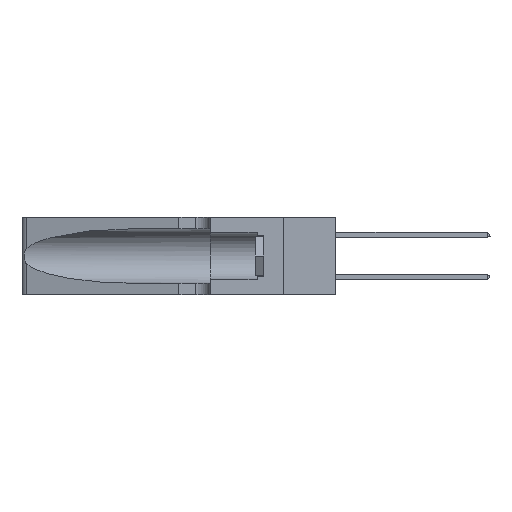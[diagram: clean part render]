
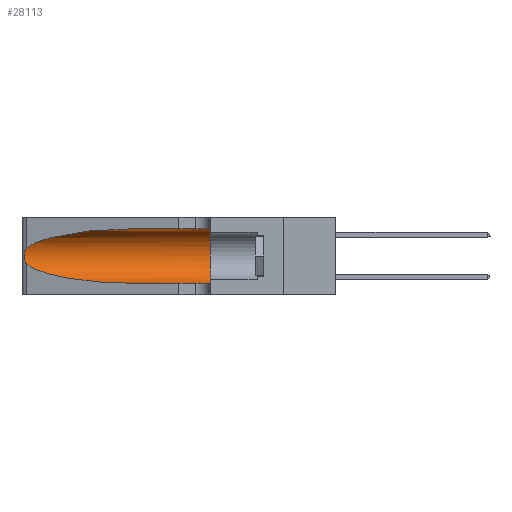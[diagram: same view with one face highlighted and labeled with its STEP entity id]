
A CAD part, left-side view. The second image highlights one B-rep face of the part: STEP entity #28113.
In plain terms, the highlighted cylindrical face has radius 3.308 mm (diameter 6.617 mm), a partial arc.
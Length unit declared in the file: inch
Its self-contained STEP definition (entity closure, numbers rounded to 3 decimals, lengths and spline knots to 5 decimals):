
#178 = CARTESIAN_POINT ( 'NONE',  ( 0.25856, 1.23593, 0.16098 ) ) ;
#697 = CARTESIAN_POINT ( 'NONE',  ( 0.1305, 0.72297, 0.05475 ) ) ;
#1665 = DIRECTION ( 'NONE',  ( 0., -1., 0. ) ) ;
#2849 = CARTESIAN_POINT ( 'NONE',  ( 0.25487, 1.22718, 0.14631 ) ) ;
#4685 = CARTESIAN_POINT ( 'NONE',  ( 0.1305, 0.35, 0.05475 ) ) ;
#5077 = CARTESIAN_POINT ( 'NONE',  ( 0.25639, 1.23186, 0.15144 ) ) ;
#5295 = CARTESIAN_POINT ( 'NONE',  ( 0.26075, 1.23896, 0.19203 ) ) ;
#5450 = ORIENTED_EDGE ( 'NONE', *, *, #28094, .T. ) ;
#5750 = CYLINDRICAL_SURFACE ( 'NONE', #9639, 0.13025 ) ;
#6101 = CARTESIAN_POINT ( 'NONE',  ( 0.25487, 1.22718, 0.22369 ) ) ;
#6136 = CARTESIAN_POINT ( 'NONE',  ( 0.2373, 1.15595, 0.08982 ) ) ;
#7564 = LINE ( 'NONE', #15028, #27845 ) ;
#8656 = DIRECTION ( 'NONE',  ( 0., 0., -1. ) ) ;
#9103 = VERTEX_POINT ( 'NONE', #15913 ) ;
#9639 = AXIS2_PLACEMENT_3D ( 'NONE', #24387, #21619, #8656 ) ;
#9834 = LINE ( 'NONE', #30056, #26365 ) ;
#10285 = VERTEX_POINT ( 'NONE', #33782 ) ;
#10960 = VERTEX_POINT ( 'NONE', #29013 ) ;
#11981 = CARTESIAN_POINT ( 'NONE',  ( 0.2373, 1.15595, 0.28018 ) ) ;
#12784 = CARTESIAN_POINT ( 'NONE',  ( 0.25555, 1.22994, 0.2215 ) ) ;
#13345 = CARTESIAN_POINT ( 'NONE',  ( 0.26018, 1.23835, 0.19895 ) ) ;
#13841 = AXIS2_PLACEMENT_3D ( 'NONE', #34091, #18221, #26415 ) ;
#15028 = CARTESIAN_POINT ( 'NONE',  ( 0.1305, 1.61858, 0.05475 ) ) ;
#15367 = ORIENTED_EDGE ( 'NONE', *, *, #23206, .T. ) ;
#15647 = CARTESIAN_POINT ( 'NONE',  ( 0.26075, 1.23896, 0.178 ) ) ;
#15913 = CARTESIAN_POINT ( 'NONE',  ( 0.1305, 0.72297, 0.05475 ) ) ;
#16049 = FACE_OUTER_BOUND ( 'NONE', #23299, .T. ) ;
#16152 = CARTESIAN_POINT ( 'NONE',  ( 0.25487, 1.22718, 0.14631 ) ) ;
#16295 = CARTESIAN_POINT ( 'NONE',  ( 0.25487, 1.22718, 0.14631 ) ) ;
#17196 = CARTESIAN_POINT ( 'NONE',  ( 0.18966, 0.96281, 0.31525 ) ) ;
#17904 = CARTESIAN_POINT ( 'NONE',  ( 0.25487, 1.22718, 0.22369 ) ) ;
#18221 = DIRECTION ( 'NONE',  ( 0., 1., 0. ) ) ;
#18653 = VERTEX_POINT ( 'NONE', #16295 ) ;
#19220 = ORIENTED_EDGE ( 'NONE', *, *, #26505, .F. ) ;
#20869 = ORIENTED_EDGE ( 'NONE', *, *, #25119, .T. ) ;
#20879 = CARTESIAN_POINT ( 'NONE',  ( 0.25854, 1.2359, 0.20912 ) ) ;
#21123 = CARTESIAN_POINT ( 'NONE',  ( 0.25789, 1.23486, 0.15765 ) ) ;
#21619 = DIRECTION ( 'NONE',  ( 0., -1., 0. ) ) ;
#21850 = CARTESIAN_POINT ( 'NONE',  ( 0.18966, 0.96281, 0.05475 ) ) ;
#23060 = ORIENTED_EDGE ( 'NONE', *, *, #26139, .T. ) ;
#23206 = EDGE_CURVE ( 'NONE', #26764, #18653, #26718, .T. ) ;
#23220 = CARTESIAN_POINT ( 'NONE',  ( 0.25787, 1.23484, 0.2124 ) ) ;
#23299 = EDGE_LOOP ( 'NONE', ( #23060, #15367, #5450, #20869, #19220, #26012 ) ) ;
#23670 = CARTESIAN_POINT ( 'NONE',  ( 0.26017, 1.23833, 0.17102 ) ) ;
#24001 = CIRCLE ( 'NONE', #13841, 0.13025 ) ;
#24387 = CARTESIAN_POINT ( 'NONE',  ( 0.1305, 1.61858, 0.185 ) ) ;
#24848 = CARTESIAN_POINT ( 'NONE',  ( 0.25487, 1.22718, 0.22369 ) ) ;
#25119 = EDGE_CURVE ( 'NONE', #9103, #27010, #7564, .T. ) ;
#25695 =( BOUNDED_CURVE ( )  B_SPLINE_CURVE ( 3, ( #16152, #6136, #21850, #697 ),
 .UNSPECIFIED., .F., .F. ) 
 B_SPLINE_CURVE_WITH_KNOTS ( ( 4, 4 ),
 ( 3.44316, 4.71239 ),
 .UNSPECIFIED. ) 
 CURVE ( )  GEOMETRIC_REPRESENTATION_ITEM ( )  RATIONAL_B_SPLINE_CURVE ( ( 1., 0.87, 0.87, 1. ) ) 
 REPRESENTATION_ITEM ( '' )  );
#26012 = ORIENTED_EDGE ( 'NONE', *, *, #28701, .F. ) ;
#26139 = EDGE_CURVE ( 'NONE', #10960, #26764, #31829, .T. ) ;
#26365 = VECTOR ( 'NONE', #27687, 39.37008 ) ;
#26415 = DIRECTION ( 'NONE',  ( 0., 0., 1. ) ) ;
#26429 = CARTESIAN_POINT ( 'NONE',  ( 0.25555, 1.22993, 0.14849 ) ) ;
#26505 = EDGE_CURVE ( 'NONE', #10285, #27010, #24001, .T. ) ;
#26718 = B_SPLINE_CURVE_WITH_KNOTS ( 'NONE', 3,
 ( #17904, #12784, #33998, #23220, #20879, #13345, #5295, #15647, #23670, #178, #21123, #5077, #26429, #2849 ),
 .UNSPECIFIED., .F., .F.,
 ( 4, 2, 2, 2, 2, 2, 4 ),
 ( 0., 0.00027, 0.00053, 0.00107, 0.0016, 0.00187, 0.00214 ),
 .UNSPECIFIED. ) ;
#26764 = VERTEX_POINT ( 'NONE', #6101 ) ;
#27010 = VERTEX_POINT ( 'NONE', #4685 ) ;
#27687 = DIRECTION ( 'NONE',  ( 0., -1., 0. ) ) ;
#27845 = VECTOR ( 'NONE', #1665, 39.37008 ) ;
#28094 = EDGE_CURVE ( 'NONE', #18653, #9103, #25695, .T. ) ;
#28113 = ADVANCED_FACE ( 'NONE', ( #16049 ), #5750, .F. ) ;
#28701 = EDGE_CURVE ( 'NONE', #10960, #10285, #9834, .T. ) ;
#29013 = CARTESIAN_POINT ( 'NONE',  ( 0.1305, 0.72297, 0.31525 ) ) ;
#30056 = CARTESIAN_POINT ( 'NONE',  ( 0.1305, 1.61858, 0.31525 ) ) ;
#30644 = CARTESIAN_POINT ( 'NONE',  ( 0.1305, 0.72297, 0.31525 ) ) ;
#31829 =( BOUNDED_CURVE ( )  B_SPLINE_CURVE ( 3, ( #30644, #17196, #11981, #24848 ),
 .UNSPECIFIED., .F., .F. ) 
 B_SPLINE_CURVE_WITH_KNOTS ( ( 4, 4 ),
 ( 1.5708, 2.84003 ),
 .UNSPECIFIED. ) 
 CURVE ( )  GEOMETRIC_REPRESENTATION_ITEM ( )  RATIONAL_B_SPLINE_CURVE ( ( 1., 0.87, 0.87, 1. ) ) 
 REPRESENTATION_ITEM ( '' )  );
#33782 = CARTESIAN_POINT ( 'NONE',  ( 0.1305, 0.35, 0.31525 ) ) ;
#33998 = CARTESIAN_POINT ( 'NONE',  ( 0.25639, 1.23184, 0.21858 ) ) ;
#34091 = CARTESIAN_POINT ( 'NONE',  ( 0.1305, 0.35, 0.185 ) ) ;
